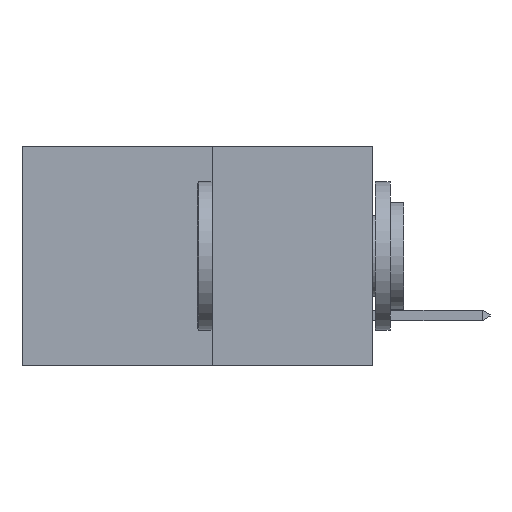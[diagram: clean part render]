
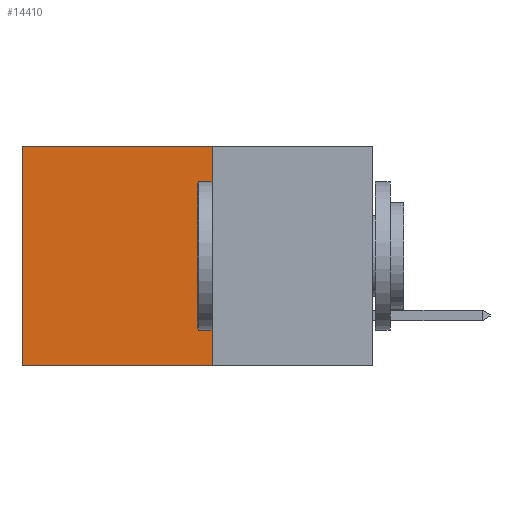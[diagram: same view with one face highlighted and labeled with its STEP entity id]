
A CAD part, left-side view. The second image highlights one B-rep face of the part: STEP entity #14410.
In plain terms, the highlighted planar face has unit normal (-1, 0, 0).
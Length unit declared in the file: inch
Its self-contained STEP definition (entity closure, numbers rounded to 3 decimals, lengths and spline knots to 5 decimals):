
#998 = FACE_OUTER_BOUND ( 'NONE', #12387, .T. ) ;
#1121 = CARTESIAN_POINT ( 'NONE',  ( 0.277, 0.27, 0. ) ) ;
#1762 = ORIENTED_EDGE ( 'NONE', *, *, #8311, .T. ) ;
#1858 = ORIENTED_EDGE ( 'NONE', *, *, #10865, .F. ) ;
#1914 = LINE ( 'NONE', #11006, #4721 ) ;
#2103 = ORIENTED_EDGE ( 'NONE', *, *, #4564, .F. ) ;
#2159 = ORIENTED_EDGE ( 'NONE', *, *, #11983, .T. ) ;
#2328 = CARTESIAN_POINT ( 'NONE',  ( 0.277, 0.27, 0. ) ) ;
#3632 = VERTEX_POINT ( 'NONE', #9192 ) ;
#4060 = VECTOR ( 'NONE', #9270, 39.37008 ) ;
#4451 = LINE ( 'NONE', #2328, #4060 ) ;
#4463 = PLANE ( 'NONE',  #13324 ) ;
#4564 = EDGE_CURVE ( 'NONE', #10615, #3632, #6801, .T. ) ;
#4629 = VECTOR ( 'NONE', #8500, 39.37008 ) ;
#4721 = VECTOR ( 'NONE', #10776, 39.37008 ) ;
#5557 = VERTEX_POINT ( 'NONE', #13762 ) ;
#6801 = LINE ( 'NONE', #14247, #7153 ) ;
#6807 = DIRECTION ( 'NONE',  ( 0., 0., -1. ) ) ;
#7153 = VECTOR ( 'NONE', #13646, 39.37008 ) ;
#8165 = CARTESIAN_POINT ( 'NONE',  ( 0.277, 0.59, -0.37 ) ) ;
#8311 = EDGE_CURVE ( 'NONE', #5557, #8869, #1914, .T. ) ;
#8500 = DIRECTION ( 'NONE',  ( 0., 1., 0. ) ) ;
#8869 = VERTEX_POINT ( 'NONE', #8165 ) ;
#9192 = CARTESIAN_POINT ( 'NONE',  ( 0.277, 0.27, -0.37 ) ) ;
#9270 = DIRECTION ( 'NONE',  ( 0., 1., 0. ) ) ;
#9636 = CARTESIAN_POINT ( 'NONE',  ( 0.277, 0.27, -0.37 ) ) ;
#10615 = VERTEX_POINT ( 'NONE', #1121 ) ;
#10776 = DIRECTION ( 'NONE',  ( 0., 0., -1. ) ) ;
#10865 = EDGE_CURVE ( 'NONE', #3632, #8869, #10950, .T. ) ;
#10950 = LINE ( 'NONE', #9636, #4629 ) ;
#11006 = CARTESIAN_POINT ( 'NONE',  ( 0.277, 0.59, -0.37 ) ) ;
#11983 = EDGE_CURVE ( 'NONE', #10615, #5557, #4451, .T. ) ;
#12276 = CARTESIAN_POINT ( 'NONE',  ( 0.277, 0.27, -0.37 ) ) ;
#12387 = EDGE_LOOP ( 'NONE', ( #1762, #1858, #2103, #2159 ) ) ;
#13324 = AXIS2_PLACEMENT_3D ( 'NONE', #12276, #13349, #6807 ) ;
#13349 = DIRECTION ( 'NONE',  ( 1., 0., 0. ) ) ;
#13646 = DIRECTION ( 'NONE',  ( 0., 0., -1. ) ) ;
#13762 = CARTESIAN_POINT ( 'NONE',  ( 0.277, 0.59, 0. ) ) ;
#14247 = CARTESIAN_POINT ( 'NONE',  ( 0.277, 0.27, -0.37 ) ) ;
#14410 = ADVANCED_FACE ( 'NONE', ( #998 ), #4463, .F. ) ;
